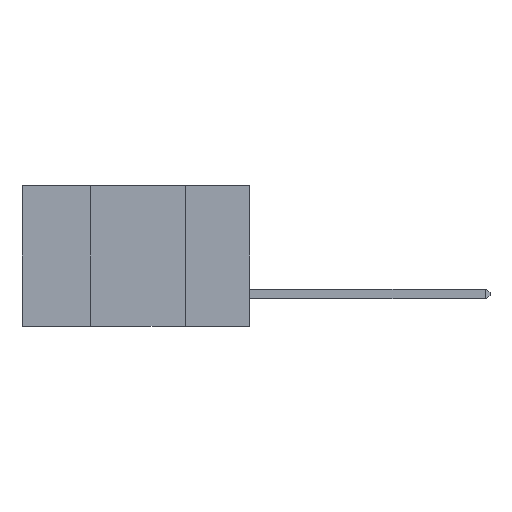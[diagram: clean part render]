
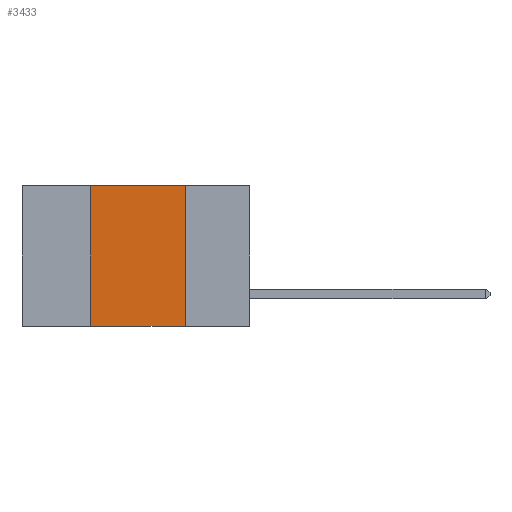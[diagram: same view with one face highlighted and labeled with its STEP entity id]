
A CAD part, left-side view. The second image highlights one B-rep face of the part: STEP entity #3433.
In plain terms, the highlighted planar face has unit normal (-1, 0, 0).
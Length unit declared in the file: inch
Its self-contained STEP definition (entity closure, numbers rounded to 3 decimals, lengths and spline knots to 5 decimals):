
#34 = DIRECTION ( 'NONE',  ( 1., 0., 0. ) ) ;
#243 = VECTOR ( 'NONE', #4893, 39.37008 ) ;
#525 = AXIS2_PLACEMENT_3D ( 'NONE', #12645, #34, #7633 ) ;
#925 = CARTESIAN_POINT ( 'NONE',  ( 0., 0.6, 0. ) ) ;
#1489 = EDGE_CURVE ( 'NONE', #9296, #6651, #6983, .T. ) ;
#1512 = VECTOR ( 'NONE', #2201, 39.37008 ) ;
#1620 = CARTESIAN_POINT ( 'NONE',  ( 0., 0.42, 0. ) ) ;
#2201 = DIRECTION ( 'NONE',  ( 0., -1., 0. ) ) ;
#2872 = CARTESIAN_POINT ( 'NONE',  ( 0., 0.17, 0. ) ) ;
#3063 = ORIENTED_EDGE ( 'NONE', *, *, #12945, .F. ) ;
#3433 = ADVANCED_FACE ( 'NONE', ( #12294 ), #5537, .F. ) ;
#3647 = CARTESIAN_POINT ( 'NONE',  ( 0., 0.42, -0.37 ) ) ;
#3840 = LINE ( 'NONE', #1620, #243 ) ;
#3965 = VECTOR ( 'NONE', #7233, 39.37008 ) ;
#4226 = VERTEX_POINT ( 'NONE', #11071 ) ;
#4833 = EDGE_LOOP ( 'NONE', ( #7598, #8742, #3063, #7930 ) ) ;
#4893 = DIRECTION ( 'NONE',  ( 0., 0., 1. ) ) ;
#5486 = CARTESIAN_POINT ( 'NONE',  ( 0., 0.6, -0.37 ) ) ;
#5537 = PLANE ( 'NONE',  #525 ) ;
#5946 = VECTOR ( 'NONE', #8453, 39.37008 ) ;
#6651 = VERTEX_POINT ( 'NONE', #13339 ) ;
#6864 = LINE ( 'NONE', #2872, #3965 ) ;
#6883 = EDGE_CURVE ( 'NONE', #4226, #6651, #6864, .T. ) ;
#6983 = LINE ( 'NONE', #5486, #1512 ) ;
#7233 = DIRECTION ( 'NONE',  ( 0., 0., -1. ) ) ;
#7598 = ORIENTED_EDGE ( 'NONE', *, *, #6883, .F. ) ;
#7633 = DIRECTION ( 'NONE',  ( 0., 0., -1. ) ) ;
#7930 = ORIENTED_EDGE ( 'NONE', *, *, #1489, .T. ) ;
#8453 = DIRECTION ( 'NONE',  ( 0., -1., 0. ) ) ;
#8709 = LINE ( 'NONE', #925, #5946 ) ;
#8742 = ORIENTED_EDGE ( 'NONE', *, *, #11157, .F. ) ;
#9296 = VERTEX_POINT ( 'NONE', #3647 ) ;
#10428 = VERTEX_POINT ( 'NONE', #10469 ) ;
#10469 = CARTESIAN_POINT ( 'NONE',  ( 0., 0.42, 0. ) ) ;
#11071 = CARTESIAN_POINT ( 'NONE',  ( 0., 0.17, 0. ) ) ;
#11157 = EDGE_CURVE ( 'NONE', #10428, #4226, #8709, .T. ) ;
#12294 = FACE_OUTER_BOUND ( 'NONE', #4833, .T. ) ;
#12645 = CARTESIAN_POINT ( 'NONE',  ( 0., 0.6, 0. ) ) ;
#12945 = EDGE_CURVE ( 'NONE', #9296, #10428, #3840, .T. ) ;
#13339 = CARTESIAN_POINT ( 'NONE',  ( 0., 0.17, -0.37 ) ) ;
